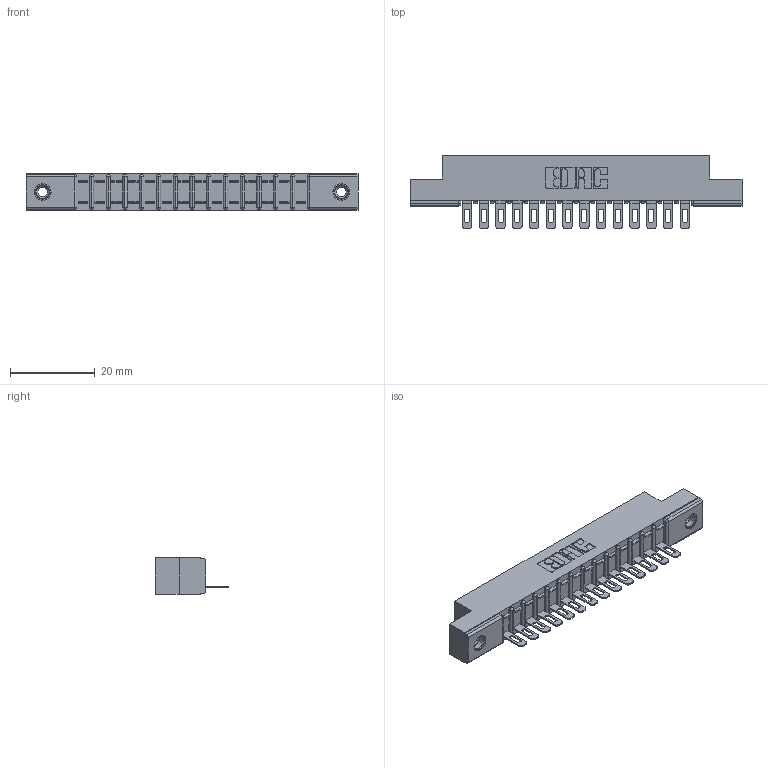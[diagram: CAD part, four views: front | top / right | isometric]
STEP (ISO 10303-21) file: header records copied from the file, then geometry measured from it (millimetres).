
FILE_DESCRIPTION (( 'STEP AP203' ), '1' );
FILE_NAME ('307-014-401-108.STEP', '2020-09-25T15:34:05', ( '' ), ( '' ), 'SwSTEP 2.0', 'SolidWorks 2020', '' );
FILE_SCHEMA (( 'CONFIG_CONTROL_DESIGN' ));
Length unit declared in the file: inch
Products named in the file (6): 345-250-001_345-250-003-102; 307 Part_.156 Dia Mounting Holes; 307-014-401-108; 307-290-002_501; #17640; #1987
Assembly tree (17 placements, depth 2):
  307-014-401-108
    307 Part_.156 Dia Mounting Holes
    307-290-002_501  x14
    345-250-001_345-250-003-102  x2
  #17640
  #1987
Bounding box: 78.49 x 17.42 x 8.71 mm (x, y, z)
Volume: 5183 mm3; surface area: 9095.1 mm2
Topology: 17 solids, 17 shells, 1257 faces, 3791 edges, 2478 vertices
Faces by surface type: plane 718, cylinder 493, sphere 30, cone 12, torus 4
Entity records: 21671 total; most frequent: ORIENTED_EDGE 3619, CARTESIAN_POINT 3609, DIRECTION 3585, EDGE_CURVE 1810, VECTOR 1359, LINE 1353, VERTEX_POINT 1150, AXIS2_PLACEMENT_3D 1094
